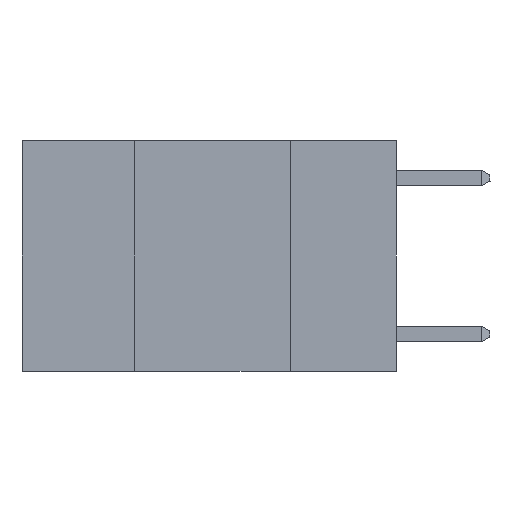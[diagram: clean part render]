
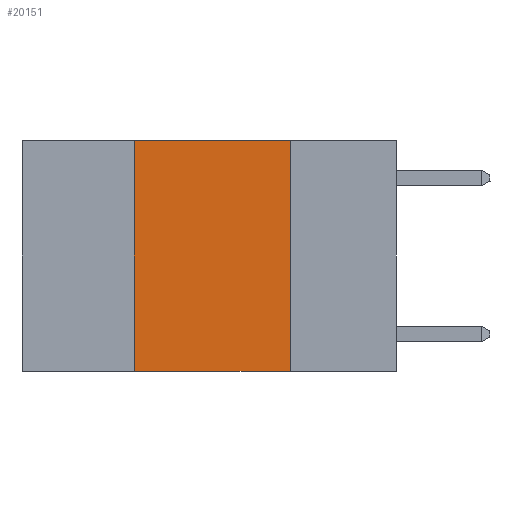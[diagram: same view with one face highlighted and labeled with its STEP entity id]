
A CAD part, left-side view. The second image highlights one B-rep face of the part: STEP entity #20151.
In plain terms, the highlighted planar face has unit normal (-1, 0, 0).
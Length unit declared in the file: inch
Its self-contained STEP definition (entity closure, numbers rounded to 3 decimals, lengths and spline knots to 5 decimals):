
#316 = LINE ( 'NONE', #17493, #14295 ) ;
#1737 = VECTOR ( 'NONE', #20368, 39.37008 ) ;
#2635 = VECTOR ( 'NONE', #20348, 39.37008 ) ;
#3240 = FACE_OUTER_BOUND ( 'NONE', #21511, .T. ) ;
#3475 = EDGE_CURVE ( 'NONE', #18062, #5076, #12264, .T. ) ;
#3729 = CARTESIAN_POINT ( 'NONE',  ( 0., 0.42, 0. ) ) ;
#3858 = CARTESIAN_POINT ( 'NONE',  ( 0., 0.17, 0. ) ) ;
#5015 = CARTESIAN_POINT ( 'NONE',  ( 0., 0.6, 0. ) ) ;
#5076 = VERTEX_POINT ( 'NONE', #3858 ) ;
#5351 = ORIENTED_EDGE ( 'NONE', *, *, #14231, .F. ) ;
#5403 = ORIENTED_EDGE ( 'NONE', *, *, #3475, .F. ) ;
#5594 = ORIENTED_EDGE ( 'NONE', *, *, #17700, .F. ) ;
#5639 = ORIENTED_EDGE ( 'NONE', *, *, #6686, .T. ) ;
#6522 = CARTESIAN_POINT ( 'NONE',  ( 0., 0.17, 0. ) ) ;
#6686 = EDGE_CURVE ( 'NONE', #13332, #16806, #316, .T. ) ;
#7103 = DIRECTION ( 'NONE',  ( 0., -1., 0. ) ) ;
#7634 = VECTOR ( 'NONE', #20609, 39.37008 ) ;
#7846 = LINE ( 'NONE', #6522, #2635 ) ;
#7889 = DIRECTION ( 'NONE',  ( 0., 0., -1. ) ) ;
#10053 = CARTESIAN_POINT ( 'NONE',  ( 0., 0.42, 0. ) ) ;
#11056 = LINE ( 'NONE', #10053, #1737 ) ;
#12264 = LINE ( 'NONE', #5015, #7634 ) ;
#13332 = VERTEX_POINT ( 'NONE', #14639 ) ;
#14231 = EDGE_CURVE ( 'NONE', #5076, #16806, #7846, .T. ) ;
#14295 = VECTOR ( 'NONE', #7103, 39.37008 ) ;
#14639 = CARTESIAN_POINT ( 'NONE',  ( 0., 0.42, -0.37 ) ) ;
#14733 = CARTESIAN_POINT ( 'NONE',  ( 0., 0.17, -0.37 ) ) ;
#14832 = CARTESIAN_POINT ( 'NONE',  ( 0., 0.6, 0. ) ) ;
#16806 = VERTEX_POINT ( 'NONE', #14733 ) ;
#17493 = CARTESIAN_POINT ( 'NONE',  ( 0., 0.6, -0.37 ) ) ;
#17700 = EDGE_CURVE ( 'NONE', #13332, #18062, #11056, .T. ) ;
#18062 = VERTEX_POINT ( 'NONE', #3729 ) ;
#18207 = PLANE ( 'NONE',  #19372 ) ;
#18274 = DIRECTION ( 'NONE',  ( 1., 0., 0. ) ) ;
#19372 = AXIS2_PLACEMENT_3D ( 'NONE', #14832, #18274, #7889 ) ;
#20151 = ADVANCED_FACE ( 'NONE', ( #3240 ), #18207, .F. ) ;
#20348 = DIRECTION ( 'NONE',  ( 0., 0., -1. ) ) ;
#20368 = DIRECTION ( 'NONE',  ( 0., 0., 1. ) ) ;
#20609 = DIRECTION ( 'NONE',  ( 0., -1., 0. ) ) ;
#21511 = EDGE_LOOP ( 'NONE', ( #5351, #5403, #5594, #5639 ) ) ;
